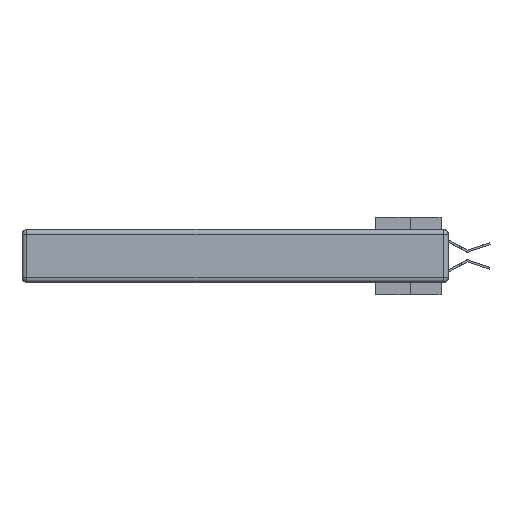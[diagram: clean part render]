
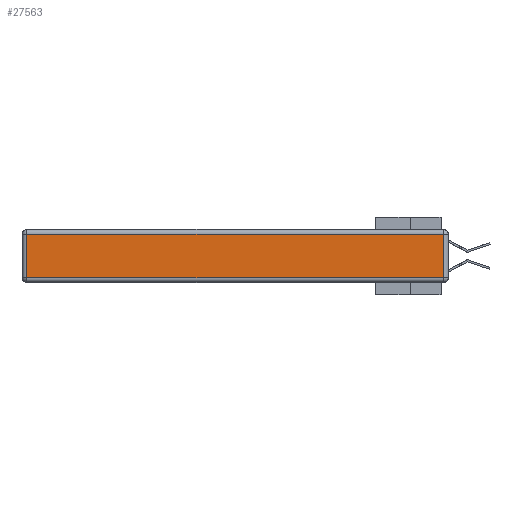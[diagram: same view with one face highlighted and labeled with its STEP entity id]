
A CAD part, left-side view. The second image highlights one B-rep face of the part: STEP entity #27563.
In plain terms, the highlighted planar face has unit normal (-1, 0, 0).
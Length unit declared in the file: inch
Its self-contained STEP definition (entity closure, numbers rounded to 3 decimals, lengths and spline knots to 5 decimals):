
#528 = LINE ( 'NONE', #25657, #10220 ) ;
#1626 = ORIENTED_EDGE ( 'NONE', *, *, #26436, .T. ) ;
#1854 = VERTEX_POINT ( 'NONE', #29625 ) ;
#3955 = DIRECTION ( 'NONE',  ( 0., 0., 1. ) ) ;
#3968 = DIRECTION ( 'NONE',  ( 0., 0., 1. ) ) ;
#4299 = CARTESIAN_POINT ( 'NONE',  ( 0., 0.03, -0.313 ) ) ;
#5735 = VERTEX_POINT ( 'NONE', #4299 ) ;
#6175 = VECTOR ( 'NONE', #14594, 39.37008 ) ;
#9265 = CARTESIAN_POINT ( 'NONE',  ( 0., 0., -0.343 ) ) ;
#9807 = FACE_OUTER_BOUND ( 'NONE', #29715, .T. ) ;
#10220 = VECTOR ( 'NONE', #25549, 39.37008 ) ;
#10257 = VECTOR ( 'NONE', #20086, 39.37008 ) ;
#12176 = CARTESIAN_POINT ( 'NONE',  ( 0., 2.72, -0.343 ) ) ;
#14594 = DIRECTION ( 'NONE',  ( 0., 0., -1. ) ) ;
#14620 = CARTESIAN_POINT ( 'NONE',  ( 0., 2.72, -0.03 ) ) ;
#14741 = CARTESIAN_POINT ( 'NONE',  ( 0., 0.03, -0.343 ) ) ;
#14773 = LINE ( 'NONE', #25082, #10257 ) ;
#16134 = VECTOR ( 'NONE', #3955, 39.37008 ) ;
#16503 = ORIENTED_EDGE ( 'NONE', *, *, #26605, .T. ) ;
#16522 = CARTESIAN_POINT ( 'NONE',  ( 0., 0.03, -0.03 ) ) ;
#16848 = ORIENTED_EDGE ( 'NONE', *, *, #26419, .T. ) ;
#19366 = VERTEX_POINT ( 'NONE', #16522 ) ;
#20086 = DIRECTION ( 'NONE',  ( 0., -1., 0. ) ) ;
#21528 = AXIS2_PLACEMENT_3D ( 'NONE', #9265, #27293, #3968 ) ;
#22133 = VERTEX_POINT ( 'NONE', #14620 ) ;
#22255 = LINE ( 'NONE', #14741, #16134 ) ;
#23723 = EDGE_CURVE ( 'NONE', #5735, #19366, #22255, .T. ) ;
#25082 = CARTESIAN_POINT ( 'NONE',  ( 0., 0., -0.313 ) ) ;
#25549 = DIRECTION ( 'NONE',  ( 0., 1., 0. ) ) ;
#25657 = CARTESIAN_POINT ( 'NONE',  ( 0., 2.75, -0.03 ) ) ;
#26419 = EDGE_CURVE ( 'NONE', #1854, #5735, #14773, .T. ) ;
#26436 = EDGE_CURVE ( 'NONE', #22133, #1854, #30291, .T. ) ;
#26605 = EDGE_CURVE ( 'NONE', #19366, #22133, #528, .T. ) ;
#27293 = DIRECTION ( 'NONE',  ( -1., 0., 0. ) ) ;
#27563 = ADVANCED_FACE ( 'NONE', ( #9807 ), #32478, .T. ) ;
#29625 = CARTESIAN_POINT ( 'NONE',  ( 0., 2.72, -0.313 ) ) ;
#29715 = EDGE_LOOP ( 'NONE', ( #16848, #30724, #16503, #1626 ) ) ;
#30291 = LINE ( 'NONE', #12176, #6175 ) ;
#30724 = ORIENTED_EDGE ( 'NONE', *, *, #23723, .T. ) ;
#32478 = PLANE ( 'NONE',  #21528 ) ;
